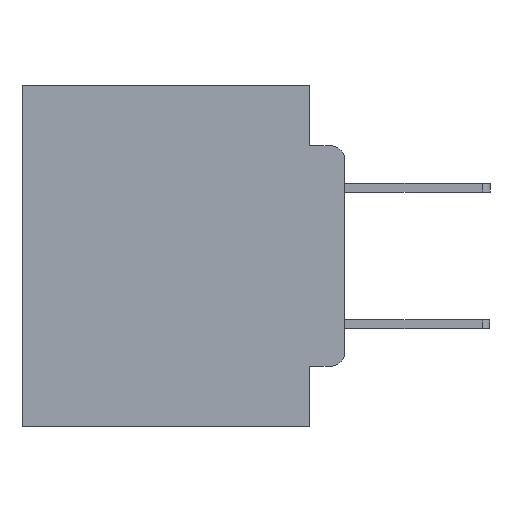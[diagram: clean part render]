
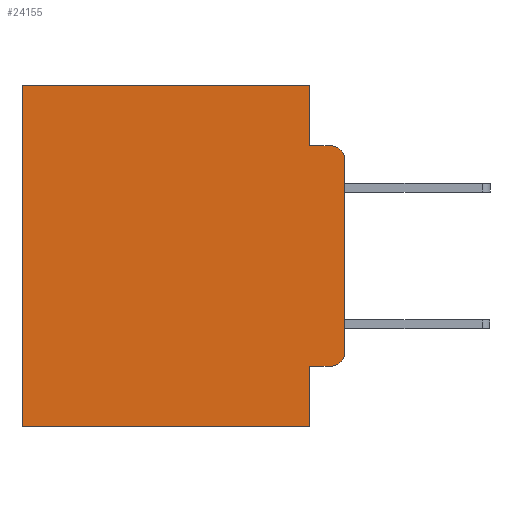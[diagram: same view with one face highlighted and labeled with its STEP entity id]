
A CAD part, left-side view. The second image highlights one B-rep face of the part: STEP entity #24155.
In plain terms, the highlighted planar face has unit normal (-1, 0, 0).
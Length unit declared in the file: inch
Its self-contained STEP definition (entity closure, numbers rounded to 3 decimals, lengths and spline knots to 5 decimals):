
#135 = DIRECTION ( 'NONE',  ( 0., 0., -1. ) ) ;
#247 = CARTESIAN_POINT ( 'NONE',  ( 0.298, 0.051, -0.0885 ) ) ;
#357 = CARTESIAN_POINT ( 'NONE',  ( 0.298, 0.051, 0. ) ) ;
#426 = ORIENTED_EDGE ( 'NONE', *, *, #20714, .T. ) ;
#669 = VERTEX_POINT ( 'NONE', #12353 ) ;
#683 = EDGE_CURVE ( 'NONE', #17596, #12329, #25449, .T. ) ;
#955 = VERTEX_POINT ( 'NONE', #25647 ) ;
#1199 = LINE ( 'NONE', #18560, #11771 ) ;
#1997 = VERTEX_POINT ( 'NONE', #13205 ) ;
#2154 = CIRCLE ( 'NONE', #20985, 0.02 ) ;
#2405 = CARTESIAN_POINT ( 'NONE',  ( 0.298, 0.02, -0.4115 ) ) ;
#2494 = DIRECTION ( 'NONE',  ( 0., 0., -1. ) ) ;
#2584 = CARTESIAN_POINT ( 'NONE',  ( 0.298, 0.051, 0. ) ) ;
#2744 = CARTESIAN_POINT ( 'NONE',  ( 0.298, 0.051, -0.5 ) ) ;
#3299 = VERTEX_POINT ( 'NONE', #2744 ) ;
#3737 = DIRECTION ( 'NONE',  ( 0., 0., -1. ) ) ;
#4919 = CARTESIAN_POINT ( 'NONE',  ( 0.298, 0.051, -0.0885 ) ) ;
#5243 = CARTESIAN_POINT ( 'NONE',  ( 0.298, 0., -0.1085 ) ) ;
#5811 = ORIENTED_EDGE ( 'NONE', *, *, #16769, .F. ) ;
#5918 = VECTOR ( 'NONE', #20571, 39.37008 ) ;
#6581 = LINE ( 'NONE', #14462, #5918 ) ;
#6632 = CARTESIAN_POINT ( 'NONE',  ( 0.298, 0.02, -0.1085 ) ) ;
#7402 = ORIENTED_EDGE ( 'NONE', *, *, #16925, .F. ) ;
#7539 = DIRECTION ( 'NONE',  ( 0., 0., -1. ) ) ;
#7722 = VERTEX_POINT ( 'NONE', #15175 ) ;
#8368 = ORIENTED_EDGE ( 'NONE', *, *, #24811, .T. ) ;
#8765 = DIRECTION ( 'NONE',  ( 0., 0., -1. ) ) ;
#9481 = FACE_OUTER_BOUND ( 'NONE', #16826, .T. ) ;
#10900 = DIRECTION ( 'NONE',  ( 0., -1., 0. ) ) ;
#10933 = AXIS2_PLACEMENT_3D ( 'NONE', #22487, #14226, #14256 ) ;
#11595 = LINE ( 'NONE', #247, #21136 ) ;
#11771 = VECTOR ( 'NONE', #20541, 39.37008 ) ;
#11911 = VERTEX_POINT ( 'NONE', #2584 ) ;
#12087 = CARTESIAN_POINT ( 'NONE',  ( 0.298, 0., 0. ) ) ;
#12329 = VERTEX_POINT ( 'NONE', #16561 ) ;
#12353 = CARTESIAN_POINT ( 'NONE',  ( 0.298, 0.051, -0.4115 ) ) ;
#12742 = DIRECTION ( 'NONE',  ( 1., 0., 0. ) ) ;
#12802 = CARTESIAN_POINT ( 'NONE',  ( 0.298, 0., -0.5 ) ) ;
#12887 = LINE ( 'NONE', #357, #23658 ) ;
#13094 = VECTOR ( 'NONE', #23000, 39.37008 ) ;
#13205 = CARTESIAN_POINT ( 'NONE',  ( 0.298, 0.473, -0.5 ) ) ;
#13242 = ORIENTED_EDGE ( 'NONE', *, *, #20803, .F. ) ;
#14226 = DIRECTION ( 'NONE',  ( -1., 0., 0. ) ) ;
#14256 = DIRECTION ( 'NONE',  ( 0., 0., -1. ) ) ;
#14454 = LINE ( 'NONE', #25813, #24532 ) ;
#14462 = CARTESIAN_POINT ( 'NONE',  ( 0.298, 0.051, 0. ) ) ;
#14597 = DIRECTION ( 'NONE',  ( 0., -1., 0. ) ) ;
#14691 = CARTESIAN_POINT ( 'NONE',  ( 0.298, 0.051, -0.4115 ) ) ;
#15175 = CARTESIAN_POINT ( 'NONE',  ( 0.298, 0.473, 0. ) ) ;
#15395 = EDGE_CURVE ( 'NONE', #7722, #1997, #14454, .T. ) ;
#15540 = EDGE_CURVE ( 'NONE', #19201, #12329, #25456, .T. ) ;
#15604 = ORIENTED_EDGE ( 'NONE', *, *, #15395, .T. ) ;
#16561 = CARTESIAN_POINT ( 'NONE',  ( 0.298, 0., -0.3915 ) ) ;
#16769 = EDGE_CURVE ( 'NONE', #11911, #23178, #6581, .T. ) ;
#16826 = EDGE_LOOP ( 'NONE', ( #19934, #8368, #13242, #5811, #21572, #15604, #7402, #17161, #426, #21826 ) ) ;
#16925 = EDGE_CURVE ( 'NONE', #3299, #1997, #18584, .T. ) ;
#17161 = ORIENTED_EDGE ( 'NONE', *, *, #26054, .F. ) ;
#17442 = EDGE_CURVE ( 'NONE', #11911, #7722, #1199, .T. ) ;
#17596 = VERTEX_POINT ( 'NONE', #2405 ) ;
#18560 = CARTESIAN_POINT ( 'NONE',  ( 0.298, 0., 0. ) ) ;
#18584 = LINE ( 'NONE', #12802, #13094 ) ;
#19201 = VERTEX_POINT ( 'NONE', #5243 ) ;
#19934 = ORIENTED_EDGE ( 'NONE', *, *, #15540, .F. ) ;
#20147 = VECTOR ( 'NONE', #3737, 39.37008 ) ;
#20541 = DIRECTION ( 'NONE',  ( 0., 1., 0. ) ) ;
#20571 = DIRECTION ( 'NONE',  ( 0., 0., -1. ) ) ;
#20683 = PLANE ( 'NONE',  #24665 ) ;
#20714 = EDGE_CURVE ( 'NONE', #669, #17596, #24902, .T. ) ;
#20803 = EDGE_CURVE ( 'NONE', #23178, #955, #11595, .T. ) ;
#20985 = AXIS2_PLACEMENT_3D ( 'NONE', #6632, #21007, #8765 ) ;
#21007 = DIRECTION ( 'NONE',  ( -1., 0., 0. ) ) ;
#21136 = VECTOR ( 'NONE', #10900, 39.37008 ) ;
#21572 = ORIENTED_EDGE ( 'NONE', *, *, #17442, .T. ) ;
#21826 = ORIENTED_EDGE ( 'NONE', *, *, #683, .T. ) ;
#22487 = CARTESIAN_POINT ( 'NONE',  ( 0.298, 0.02, -0.3915 ) ) ;
#22758 = CARTESIAN_POINT ( 'NONE',  ( 0.298, 0., 0. ) ) ;
#23000 = DIRECTION ( 'NONE',  ( 0., 1., 0. ) ) ;
#23178 = VERTEX_POINT ( 'NONE', #4919 ) ;
#23644 = VECTOR ( 'NONE', #14597, 39.37008 ) ;
#23658 = VECTOR ( 'NONE', #2494, 39.37008 ) ;
#24155 = ADVANCED_FACE ( 'NONE', ( #9481 ), #20683, .F. ) ;
#24532 = VECTOR ( 'NONE', #7539, 39.37008 ) ;
#24665 = AXIS2_PLACEMENT_3D ( 'NONE', #22758, #12742, #135 ) ;
#24811 = EDGE_CURVE ( 'NONE', #19201, #955, #2154, .T. ) ;
#24902 = LINE ( 'NONE', #14691, #23644 ) ;
#25449 = CIRCLE ( 'NONE', #10933, 0.02 ) ;
#25456 = LINE ( 'NONE', #12087, #20147 ) ;
#25647 = CARTESIAN_POINT ( 'NONE',  ( 0.298, 0.02, -0.0885 ) ) ;
#25813 = CARTESIAN_POINT ( 'NONE',  ( 0.298, 0.473, 0. ) ) ;
#26054 = EDGE_CURVE ( 'NONE', #669, #3299, #12887, .T. ) ;
